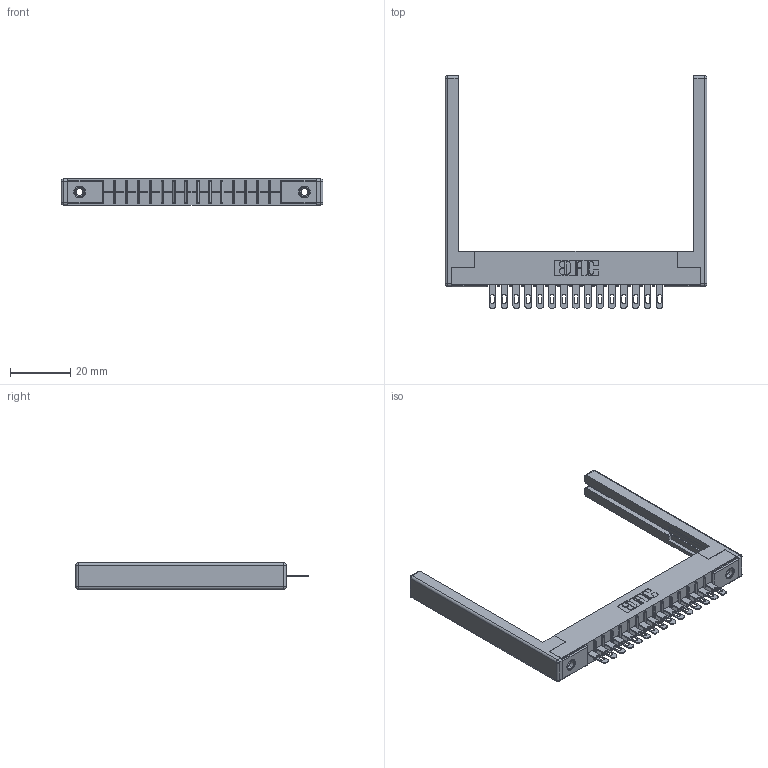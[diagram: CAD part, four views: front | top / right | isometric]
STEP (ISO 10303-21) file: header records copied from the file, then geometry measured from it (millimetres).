
FILE_DESCRIPTION (( 'STEP AP203' ), '1' );
FILE_NAME ('356-015-400-168.STEP', '2020-09-23T12:02:18', ( '' ), ( '' ), 'SwSTEP 2.0', 'SolidWorks 2020', '' );
FILE_SCHEMA (( 'CONFIG_CONTROL_DESIGN' ));
Length unit declared in the file: inch
Products named in the file (5): 356-015-400-168; 307-220-068; 345-250-001_345-250-001-102; 306-290-001_100; 306 Part_.156 Dia
Assembly tree (20 placements, depth 2):
  356-015-400-168
    306 Part_.156 Dia
    306-290-001_100  x15
    345-250-001_345-250-001-102  x2
    307-220-068  x2
Bounding box: 86.87 x 77.17 x 8.71 mm (x, y, z)
Volume: 10502.8 mm3; surface area: 12943.7 mm2
Topology: 20 solids, 20 shells, 1410 faces, 3931 edges, 2518 vertices
Faces by surface type: plane 906, cylinder 420, sphere 68, cone 12, torus 4
Entity records: 20409 total; most frequent: CARTESIAN_POINT 3389, DIRECTION 3358, ORIENTED_EDGE 3348, EDGE_CURVE 1674, LINE 1288, VECTOR 1288, VERTEX_POINT 1066, AXIS2_PLACEMENT_3D 1035
